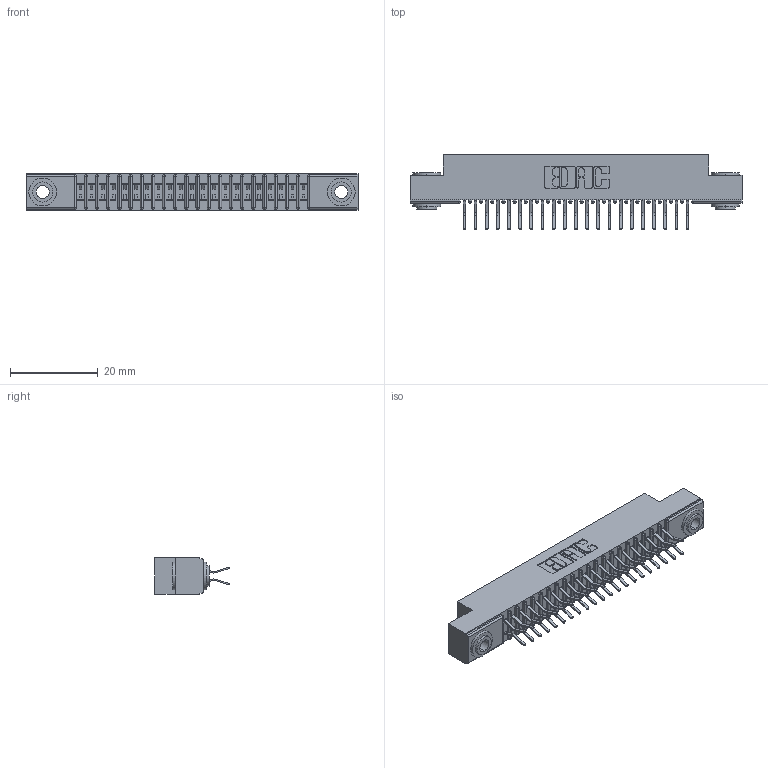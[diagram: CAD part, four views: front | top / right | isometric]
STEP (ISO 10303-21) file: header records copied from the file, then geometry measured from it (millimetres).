
FILE_DESCRIPTION (( 'STEP AP203' ), '1' );
FILE_NAME ('391-042-556-203.STEP', '2018-08-09T01:54:25', ( '' ), ( '' ), 'SwSTEP 2.0', 'SolidWorks 2016', '' );
FILE_SCHEMA (( 'CONFIG_CONTROL_DESIGN' ));
Length unit declared in the file: inch
Products named in the file (4): 391-042-556-203; 341 Part_.156 (3.96) Dia Mounting Holes; 341-292-001_341-292-156; 345-250-002_345-250-002-102
Assembly tree (45 placements, depth 2):
  391-042-556-203
    341 Part_.156 (3.96) Dia Mounting Holes
    341-292-001_341-292-156  x42
    345-250-002_345-250-002-102  x2
Bounding box: 75.56 x 17.07 x 8.38 mm (x, y, z)
Volume: 4319.4 mm3; surface area: 9274.9 mm2
Topology: 45 solids, 45 shells, 3108 faces, 8975 edges, 5822 vertices
Faces by surface type: plane 1772, cylinder 1244, sphere 44, torus 40, cone 8
Entity records: 29417 total; most frequent: CARTESIAN_POINT 4872, ORIENTED_EDGE 4830, DIRECTION 4763, EDGE_CURVE 2415, LINE 1913, VECTOR 1913, VERTEX_POINT 1534, AXIS2_PLACEMENT_3D 1425
